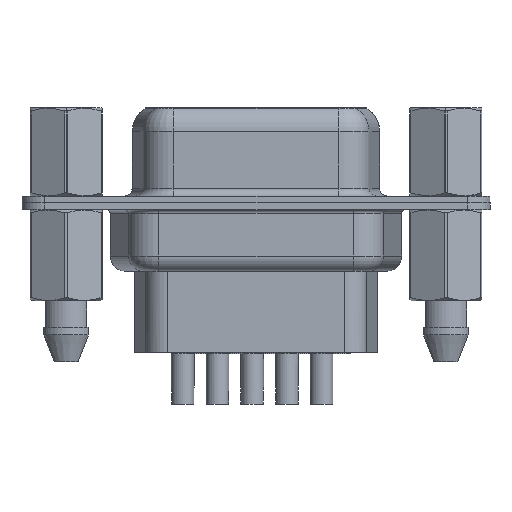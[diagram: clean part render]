
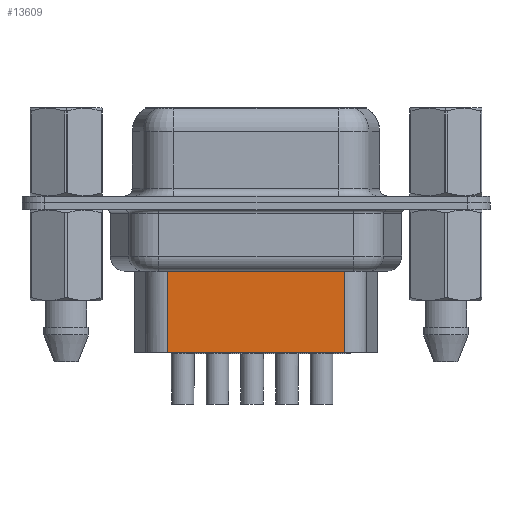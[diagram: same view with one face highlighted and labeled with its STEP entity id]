
A CAD part, front view. The second image highlights one B-rep face of the part: STEP entity #13609.
In plain terms, the highlighted planar face has unit normal (0, -1, 0).
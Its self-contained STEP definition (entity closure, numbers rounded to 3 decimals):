
#53 = PLANE ( 'NONE',  #27301 ) ;
#76 = ORIENTED_EDGE ( 'NONE', *, *, #27853, .F. ) ;
#2380 = DIRECTION ( 'NONE',  ( 1., 0., 0. ) ) ;
#3164 = EDGE_LOOP ( 'NONE', ( #27150, #4967, #17423, #76 ) ) ;
#3712 = VERTEX_POINT ( 'NONE', #22241 ) ;
#4967 = ORIENTED_EDGE ( 'NONE', *, *, #29104, .T. ) ;
#5478 = CARTESIAN_POINT ( 'NONE',  ( 6.701, -3.5, -3.1 ) ) ;
#5990 = CARTESIAN_POINT ( 'NONE',  ( 6.701, -3.5, -4.097 ) ) ;
#7399 = EDGE_CURVE ( 'NONE', #23975, #12429, #16180, .T. ) ;
#8058 = VECTOR ( 'NONE', #26728, 1000. ) ;
#8068 = CARTESIAN_POINT ( 'NONE',  ( 18.289, -3.5, -4.097 ) ) ;
#8734 = LINE ( 'NONE', #17745, #20642 ) ;
#9407 = VERTEX_POINT ( 'NONE', #8068 ) ;
#12429 = VERTEX_POINT ( 'NONE', #19651 ) ;
#12505 = CARTESIAN_POINT ( 'NONE',  ( 6.701, -3.5, -9.85 ) ) ;
#13404 = VECTOR ( 'NONE', #22092, 1000. ) ;
#13609 = ADVANCED_FACE ( 'NONE', ( #29695 ), #53, .T. ) ;
#14334 = LINE ( 'NONE', #12505, #8058 ) ;
#16180 = LINE ( 'NONE', #5478, #16927 ) ;
#16472 = DIRECTION ( 'NONE',  ( 0., -1., 0. ) ) ;
#16927 = VECTOR ( 'NONE', #19638, 1000. ) ;
#17358 = EDGE_CURVE ( 'NONE', #9407, #3712, #26067, .T. ) ;
#17423 = ORIENTED_EDGE ( 'NONE', *, *, #7399, .T. ) ;
#17745 = CARTESIAN_POINT ( 'NONE',  ( 6.454, -3.5, -4.097 ) ) ;
#19638 = DIRECTION ( 'NONE',  ( 0., 0., -1. ) ) ;
#19651 = CARTESIAN_POINT ( 'NONE',  ( 6.701, -3.5, -9.85 ) ) ;
#19662 = CARTESIAN_POINT ( 'NONE',  ( 18.289, -3.5, -3.1 ) ) ;
#20642 = VECTOR ( 'NONE', #24821, 1000. ) ;
#22092 = DIRECTION ( 'NONE',  ( 0., 0., -1. ) ) ;
#22241 = CARTESIAN_POINT ( 'NONE',  ( 18.289, -3.5, -9.85 ) ) ;
#23975 = VERTEX_POINT ( 'NONE', #5990 ) ;
#24821 = DIRECTION ( 'NONE',  ( -1., 0., 0. ) ) ;
#25911 = CARTESIAN_POINT ( 'NONE',  ( 6.701, -3.5, -3.1 ) ) ;
#26067 = LINE ( 'NONE', #19662, #13404 ) ;
#26728 = DIRECTION ( 'NONE',  ( -1., 0., 0. ) ) ;
#27150 = ORIENTED_EDGE ( 'NONE', *, *, #17358, .F. ) ;
#27301 = AXIS2_PLACEMENT_3D ( 'NONE', #25911, #16472, #2380 ) ;
#27853 = EDGE_CURVE ( 'NONE', #3712, #12429, #14334, .T. ) ;
#29104 = EDGE_CURVE ( 'NONE', #9407, #23975, #8734, .T. ) ;
#29695 = FACE_OUTER_BOUND ( 'NONE', #3164, .T. ) ;
